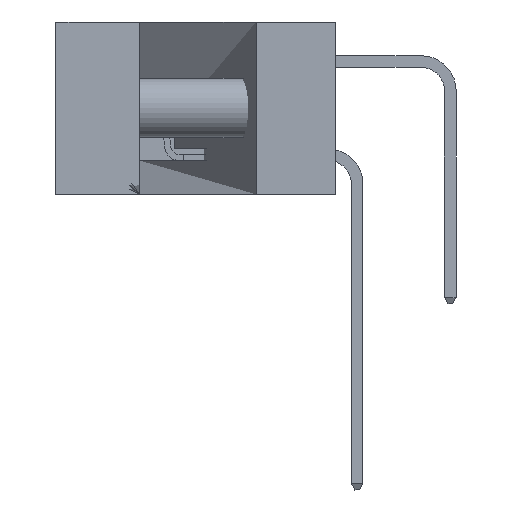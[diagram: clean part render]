
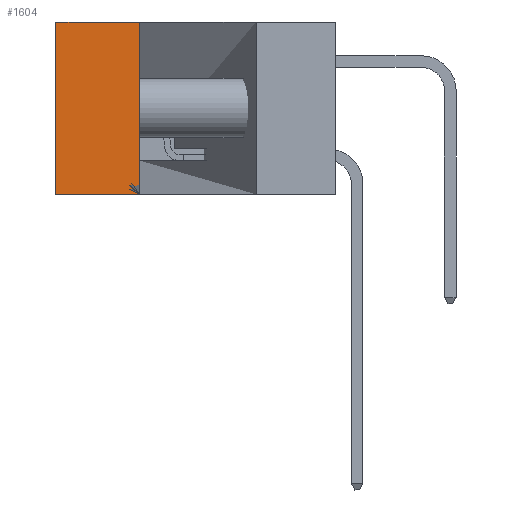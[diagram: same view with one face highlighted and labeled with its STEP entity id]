
A CAD part, left-side view. The second image highlights one B-rep face of the part: STEP entity #1604.
In plain terms, the highlighted planar face has unit normal (-1, 0, 0).
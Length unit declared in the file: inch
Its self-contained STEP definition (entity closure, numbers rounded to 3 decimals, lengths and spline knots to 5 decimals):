
#1604 = ADVANCED_FACE ( 'NONE', ( #3369 ), #24892, .F. ) ;
#2005 = DIRECTION ( 'NONE',  ( 0., 0., -1. ) ) ;
#2926 = CARTESIAN_POINT ( 'NONE',  ( 0.2875, 0.42, 0. ) ) ;
#3369 = FACE_OUTER_BOUND ( 'NONE', #6566, .T. ) ;
#3706 = DIRECTION ( 'NONE',  ( 1., 0., 0. ) ) ;
#6566 = EDGE_LOOP ( 'NONE', ( #34531, #42092, #42497, #39338 ) ) ;
#7621 = DIRECTION ( 'NONE',  ( 0., 0., -1. ) ) ;
#9467 = VERTEX_POINT ( 'NONE', #34617 ) ;
#10670 = CARTESIAN_POINT ( 'NONE',  ( 0.2875, 0.42, 0. ) ) ;
#11127 = CARTESIAN_POINT ( 'NONE',  ( 0.2875, 0.42, 0. ) ) ;
#11801 = CARTESIAN_POINT ( 'NONE',  ( 0.2875, 0.6, 0. ) ) ;
#15035 = DIRECTION ( 'NONE',  ( 0., 1., 0. ) ) ;
#16993 = VECTOR ( 'NONE', #15035, 39.37008 ) ;
#18867 = EDGE_CURVE ( 'NONE', #9467, #43974, #26178, .T. ) ;
#22037 = CARTESIAN_POINT ( 'NONE',  ( 0.2875, 0.42, -0.37 ) ) ;
#22613 = LINE ( 'NONE', #2926, #33046 ) ;
#24832 = VECTOR ( 'NONE', #2005, 39.37008 ) ;
#24892 = PLANE ( 'NONE',  #31606 ) ;
#26178 = LINE ( 'NONE', #11127, #35532 ) ;
#26356 = LINE ( 'NONE', #22037, #16993 ) ;
#26760 = CARTESIAN_POINT ( 'NONE',  ( 0.2875, 0.6, 0. ) ) ;
#27641 = DIRECTION ( 'NONE',  ( 0., 1., 0. ) ) ;
#28428 = DIRECTION ( 'NONE',  ( 0., 0., -1. ) ) ;
#31606 = AXIS2_PLACEMENT_3D ( 'NONE', #10670, #3706, #28428 ) ;
#33046 = VECTOR ( 'NONE', #27641, 39.37008 ) ;
#33082 = LINE ( 'NONE', #26760, #24832 ) ;
#33269 = VERTEX_POINT ( 'NONE', #11801 ) ;
#34011 = EDGE_CURVE ( 'NONE', #33269, #44385, #33082, .T. ) ;
#34531 = ORIENTED_EDGE ( 'NONE', *, *, #34011, .T. ) ;
#34617 = CARTESIAN_POINT ( 'NONE',  ( 0.2875, 0.42, 0. ) ) ;
#35532 = VECTOR ( 'NONE', #7621, 39.37008 ) ;
#38482 = CARTESIAN_POINT ( 'NONE',  ( 0.2875, 0.42, -0.37 ) ) ;
#39338 = ORIENTED_EDGE ( 'NONE', *, *, #44567, .T. ) ;
#42092 = ORIENTED_EDGE ( 'NONE', *, *, #45548, .F. ) ;
#42497 = ORIENTED_EDGE ( 'NONE', *, *, #18867, .F. ) ;
#43974 = VERTEX_POINT ( 'NONE', #38482 ) ;
#44190 = CARTESIAN_POINT ( 'NONE',  ( 0.2875, 0.6, -0.37 ) ) ;
#44385 = VERTEX_POINT ( 'NONE', #44190 ) ;
#44567 = EDGE_CURVE ( 'NONE', #9467, #33269, #22613, .T. ) ;
#45548 = EDGE_CURVE ( 'NONE', #43974, #44385, #26356, .T. ) ;
